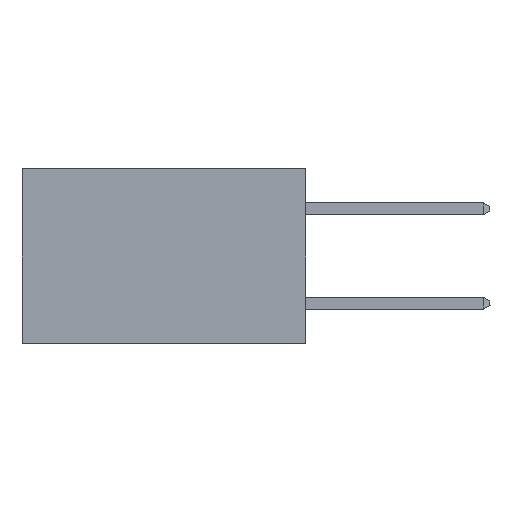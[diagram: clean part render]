
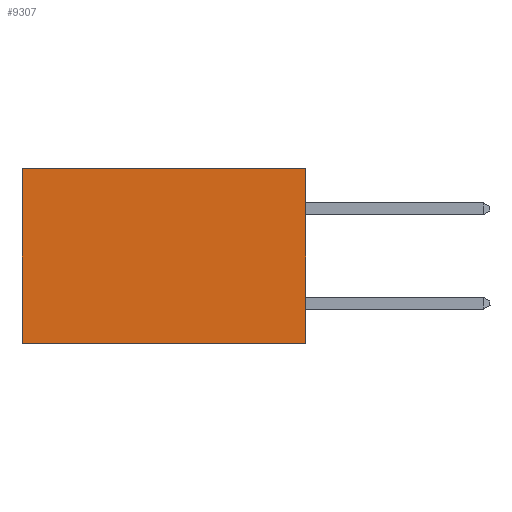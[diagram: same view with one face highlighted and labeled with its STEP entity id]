
A CAD part, left-side view. The second image highlights one B-rep face of the part: STEP entity #9307.
In plain terms, the highlighted planar face has unit normal (-1, 0, 0).
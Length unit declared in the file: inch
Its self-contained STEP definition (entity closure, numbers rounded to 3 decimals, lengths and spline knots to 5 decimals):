
#323 = DIRECTION ( 'NONE',  ( 1., 0., 0. ) ) ;
#829 = CARTESIAN_POINT ( 'NONE',  ( 0.2615, 0.6, 0. ) ) ;
#1257 = EDGE_CURVE ( 'NONE', #5904, #8238, #7231, .T. ) ;
#2221 = ORIENTED_EDGE ( 'NONE', *, *, #1257, .T. ) ;
#2291 = DIRECTION ( 'NONE',  ( 0., 1., 0. ) ) ;
#2575 = EDGE_CURVE ( 'NONE', #5219, #7752, #2771, .T. ) ;
#2771 = LINE ( 'NONE', #7408, #5502 ) ;
#3300 = ORIENTED_EDGE ( 'NONE', *, *, #9342, .F. ) ;
#3369 = PLANE ( 'NONE',  #7443 ) ;
#3395 = VECTOR ( 'NONE', #2291, 39.37008 ) ;
#3956 = DIRECTION ( 'NONE',  ( 0., 0., -1. ) ) ;
#4470 = CARTESIAN_POINT ( 'NONE',  ( 0.2615, 0., -0.37 ) ) ;
#4563 = DIRECTION ( 'NONE',  ( 0., 0., -1. ) ) ;
#5170 = VECTOR ( 'NONE', #4563, 39.37008 ) ;
#5219 = VERTEX_POINT ( 'NONE', #7868 ) ;
#5393 = CARTESIAN_POINT ( 'NONE',  ( 0.2615, 0., 0. ) ) ;
#5433 = CARTESIAN_POINT ( 'NONE',  ( 0.2615, 0.6, -0.37 ) ) ;
#5502 = VECTOR ( 'NONE', #8090, 39.37008 ) ;
#5562 = LINE ( 'NONE', #7771, #9599 ) ;
#5593 = ORIENTED_EDGE ( 'NONE', *, *, #2575, .F. ) ;
#5904 = VERTEX_POINT ( 'NONE', #5393 ) ;
#6093 = CARTESIAN_POINT ( 'NONE',  ( 0.2615, 0., 0. ) ) ;
#6126 = EDGE_LOOP ( 'NONE', ( #8181, #5593, #3300, #2221 ) ) ;
#6240 = CARTESIAN_POINT ( 'NONE',  ( 0.2615, 0., -0.37 ) ) ;
#6605 = LINE ( 'NONE', #4470, #5170 ) ;
#6838 = FACE_OUTER_BOUND ( 'NONE', #6126, .T. ) ;
#7231 = LINE ( 'NONE', #6093, #3395 ) ;
#7350 = EDGE_CURVE ( 'NONE', #8238, #7752, #5562, .T. ) ;
#7408 = CARTESIAN_POINT ( 'NONE',  ( 0.2615, 0., -0.37 ) ) ;
#7443 = AXIS2_PLACEMENT_3D ( 'NONE', #6240, #323, #8935 ) ;
#7752 = VERTEX_POINT ( 'NONE', #5433 ) ;
#7771 = CARTESIAN_POINT ( 'NONE',  ( 0.2615, 0.6, -0.37 ) ) ;
#7868 = CARTESIAN_POINT ( 'NONE',  ( 0.2615, 0., -0.37 ) ) ;
#8090 = DIRECTION ( 'NONE',  ( 0., 1., 0. ) ) ;
#8181 = ORIENTED_EDGE ( 'NONE', *, *, #7350, .T. ) ;
#8238 = VERTEX_POINT ( 'NONE', #829 ) ;
#8935 = DIRECTION ( 'NONE',  ( 0., 0., -1. ) ) ;
#9307 = ADVANCED_FACE ( 'NONE', ( #6838 ), #3369, .F. ) ;
#9342 = EDGE_CURVE ( 'NONE', #5904, #5219, #6605, .T. ) ;
#9599 = VECTOR ( 'NONE', #3956, 39.37008 ) ;
